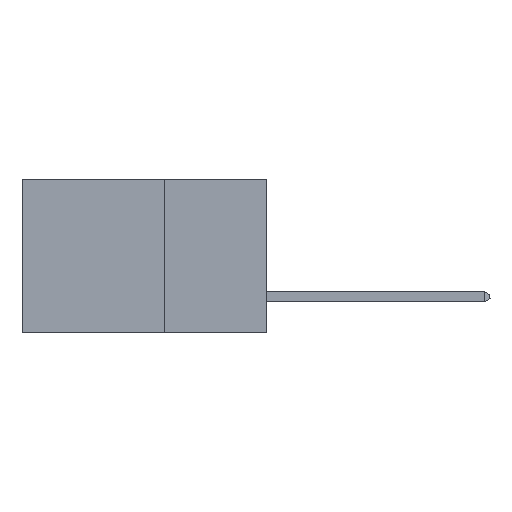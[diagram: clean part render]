
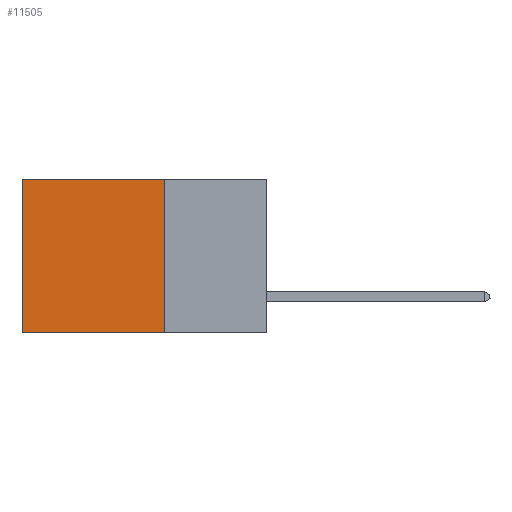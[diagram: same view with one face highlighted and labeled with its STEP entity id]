
A CAD part, left-side view. The second image highlights one B-rep face of the part: STEP entity #11505.
In plain terms, the highlighted planar face has unit normal (-1, 0, 0).
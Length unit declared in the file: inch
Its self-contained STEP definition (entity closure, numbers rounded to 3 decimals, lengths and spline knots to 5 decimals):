
#222 = VERTEX_POINT ( 'NONE', #10203 ) ;
#501 = CARTESIAN_POINT ( 'NONE',  ( 0.2875, 0.25, -0.375 ) ) ;
#523 = CARTESIAN_POINT ( 'NONE',  ( 0.2875, 0.6, -0.375 ) ) ;
#590 = ORIENTED_EDGE ( 'NONE', *, *, #1721, .F. ) ;
#602 = LINE ( 'NONE', #4676, #5458 ) ;
#689 = CARTESIAN_POINT ( 'NONE',  ( 0.2875, 0.25, 0. ) ) ;
#755 = ORIENTED_EDGE ( 'NONE', *, *, #1729, .F. ) ;
#1721 = EDGE_CURVE ( 'NONE', #4617, #2260, #602, .T. ) ;
#1723 = LINE ( 'NONE', #2664, #2043 ) ;
#1729 = EDGE_CURVE ( 'NONE', #2260, #222, #1723, .T. ) ;
#1913 = VECTOR ( 'NONE', #4596, 39.37008 ) ;
#1927 = VECTOR ( 'NONE', #10636, 39.37008 ) ;
#2043 = VECTOR ( 'NONE', #6727, 39.37008 ) ;
#2260 = VERTEX_POINT ( 'NONE', #10980 ) ;
#2471 = EDGE_LOOP ( 'NONE', ( #3966, #755, #590, #11605 ) ) ;
#2664 = CARTESIAN_POINT ( 'NONE',  ( 0.2875, 0.25, -0.375 ) ) ;
#3078 = CARTESIAN_POINT ( 'NONE',  ( 0.2875, 0.25, 0. ) ) ;
#3433 = DIRECTION ( 'NONE',  ( 1., 0., 0. ) ) ;
#3499 = FACE_OUTER_BOUND ( 'NONE', #2471, .T. ) ;
#3966 = ORIENTED_EDGE ( 'NONE', *, *, #6166, .T. ) ;
#4596 = DIRECTION ( 'NONE',  ( 0., 0., -1. ) ) ;
#4617 = VERTEX_POINT ( 'NONE', #3078 ) ;
#4659 = LINE ( 'NONE', #523, #1913 ) ;
#4676 = CARTESIAN_POINT ( 'NONE',  ( 0.2875, 0.25, -0.375 ) ) ;
#5458 = VECTOR ( 'NONE', #12803, 39.37008 ) ;
#5750 = LINE ( 'NONE', #689, #1927 ) ;
#6166 = EDGE_CURVE ( 'NONE', #7209, #222, #4659, .T. ) ;
#6727 = DIRECTION ( 'NONE',  ( 0., 1., 0. ) ) ;
#7037 = EDGE_CURVE ( 'NONE', #4617, #7209, #5750, .T. ) ;
#7209 = VERTEX_POINT ( 'NONE', #12718 ) ;
#7439 = DIRECTION ( 'NONE',  ( 0., 0., -1. ) ) ;
#8252 = AXIS2_PLACEMENT_3D ( 'NONE', #501, #3433, #7439 ) ;
#9598 = PLANE ( 'NONE',  #8252 ) ;
#10203 = CARTESIAN_POINT ( 'NONE',  ( 0.2875, 0.6, -0.375 ) ) ;
#10636 = DIRECTION ( 'NONE',  ( 0., 1., 0. ) ) ;
#10980 = CARTESIAN_POINT ( 'NONE',  ( 0.2875, 0.25, -0.375 ) ) ;
#11505 = ADVANCED_FACE ( 'NONE', ( #3499 ), #9598, .F. ) ;
#11605 = ORIENTED_EDGE ( 'NONE', *, *, #7037, .T. ) ;
#12718 = CARTESIAN_POINT ( 'NONE',  ( 0.2875, 0.6, 0. ) ) ;
#12803 = DIRECTION ( 'NONE',  ( 0., 0., -1. ) ) ;
